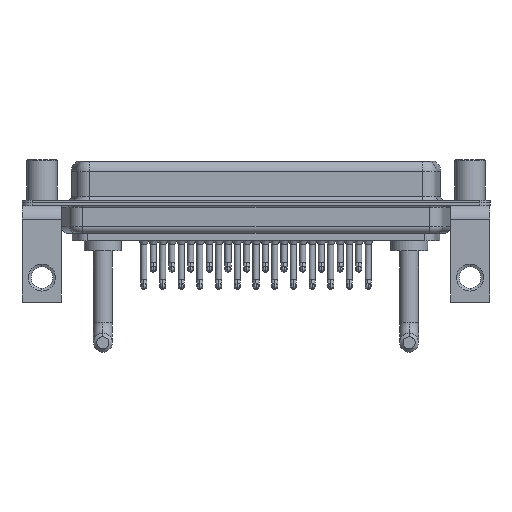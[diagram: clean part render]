
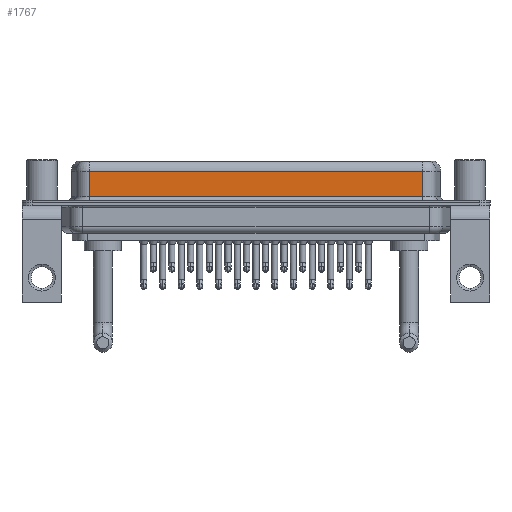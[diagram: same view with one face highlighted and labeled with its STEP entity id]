
A CAD part, front view. The second image highlights one B-rep face of the part: STEP entity #1767.
In plain terms, the highlighted planar face has unit normal (0, -1, 0).
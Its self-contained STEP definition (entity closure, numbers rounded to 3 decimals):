
#339 = DIRECTION ( 'NONE',  ( -1., 0., 0. ) ) ;
#396 = DIRECTION ( 'NONE',  ( 0., 0., -1. ) ) ;
#1194 = ORIENTED_EDGE ( 'NONE', *, *, #7303, .F. ) ;
#1767 = ADVANCED_FACE ( 'NONE', ( #11543 ), #26099, .F. ) ;
#1846 = DIRECTION ( 'NONE',  ( 0., 0., -1. ) ) ;
#3272 = VECTOR ( 'NONE', #25423, 1000. ) ;
#3355 = EDGE_LOOP ( 'NONE', ( #1194, #10700, #20481, #22734 ) ) ;
#4385 = LINE ( 'NONE', #8518, #3272 ) ;
#7121 = CARTESIAN_POINT ( 'NONE',  ( 56.462, -3.95, 6.4 ) ) ;
#7303 = EDGE_CURVE ( 'NONE', #17673, #20828, #17152, .T. ) ;
#8518 = CARTESIAN_POINT ( 'NONE',  ( 56.462, -3.95, 0.9 ) ) ;
#8609 = CARTESIAN_POINT ( 'NONE',  ( 56.462, -3.95, 4.65 ) ) ;
#8666 = CARTESIAN_POINT ( 'NONE',  ( 7.038, -3.95, 6.4 ) ) ;
#9632 = CARTESIAN_POINT ( 'NONE',  ( 7.038, -3.95, 0.9 ) ) ;
#10700 = ORIENTED_EDGE ( 'NONE', *, *, #23160, .T. ) ;
#11543 = FACE_OUTER_BOUND ( 'NONE', #3355, .T. ) ;
#12111 = VECTOR ( 'NONE', #396, 1000. ) ;
#14360 = CARTESIAN_POINT ( 'NONE',  ( 56.462, -3.95, 6.4 ) ) ;
#14679 = LINE ( 'NONE', #8609, #24013 ) ;
#14741 = LINE ( 'NONE', #8666, #12111 ) ;
#15545 = DIRECTION ( 'NONE',  ( 0., 1., 0. ) ) ;
#15574 = VERTEX_POINT ( 'NONE', #9632 ) ;
#15830 = DIRECTION ( 'NONE',  ( 0., 0., 1. ) ) ;
#15930 = CARTESIAN_POINT ( 'NONE',  ( 7.038, -3.95, 4.65 ) ) ;
#17152 = LINE ( 'NONE', #14360, #25950 ) ;
#17673 = VERTEX_POINT ( 'NONE', #23978 ) ;
#17972 = CARTESIAN_POINT ( 'NONE',  ( 56.462, -3.95, 0.9 ) ) ;
#20481 = ORIENTED_EDGE ( 'NONE', *, *, #25589, .T. ) ;
#20828 = VERTEX_POINT ( 'NONE', #17972 ) ;
#22684 = AXIS2_PLACEMENT_3D ( 'NONE', #7121, #15545, #15830 ) ;
#22734 = ORIENTED_EDGE ( 'NONE', *, *, #22854, .T. ) ;
#22854 = EDGE_CURVE ( 'NONE', #15574, #20828, #4385, .T. ) ;
#23160 = EDGE_CURVE ( 'NONE', #17673, #23376, #14679, .T. ) ;
#23376 = VERTEX_POINT ( 'NONE', #15930 ) ;
#23978 = CARTESIAN_POINT ( 'NONE',  ( 56.462, -3.95, 4.65 ) ) ;
#24013 = VECTOR ( 'NONE', #339, 1000. ) ;
#25423 = DIRECTION ( 'NONE',  ( 1., 0., 0. ) ) ;
#25589 = EDGE_CURVE ( 'NONE', #23376, #15574, #14741, .T. ) ;
#25950 = VECTOR ( 'NONE', #1846, 1000. ) ;
#26099 = PLANE ( 'NONE',  #22684 ) ;
